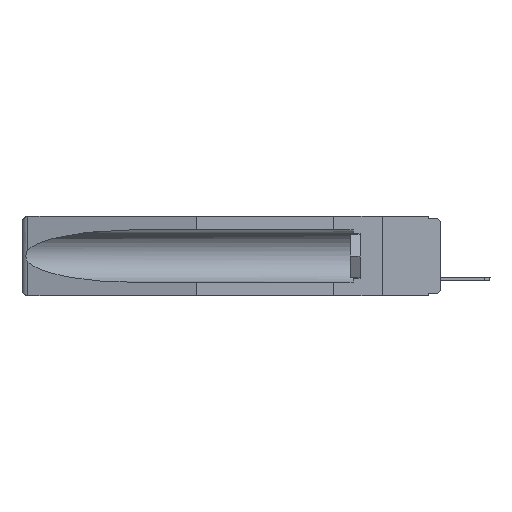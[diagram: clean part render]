
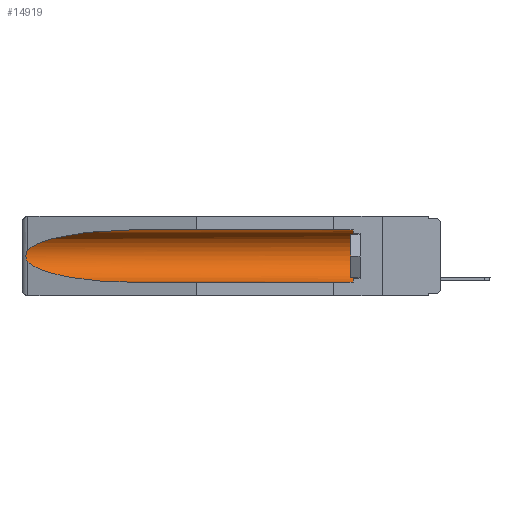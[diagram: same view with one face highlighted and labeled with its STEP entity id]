
A CAD part, left-side view. The second image highlights one B-rep face of the part: STEP entity #14919.
In plain terms, the highlighted cylindrical face has radius 2.857 mm (diameter 5.715 mm), a partial arc.
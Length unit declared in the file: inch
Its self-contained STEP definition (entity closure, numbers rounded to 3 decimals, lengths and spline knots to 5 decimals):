
#350 = DIRECTION ( 'NONE',  ( 0., 1., 0. ) ) ;
#384 = CARTESIAN_POINT ( 'NONE',  ( 0.155, 1.07973, -0.059 ) ) ;
#424 = ORIENTED_EDGE ( 'NONE', *, *, #5626, .T. ) ;
#513 = VERTEX_POINT ( 'NONE', #18364 ) ;
#762 = ORIENTED_EDGE ( 'NONE', *, *, #15672, .F. ) ;
#1241 = VECTOR ( 'NONE', #18341, 39.37008 ) ;
#1382 = VERTEX_POINT ( 'NONE', #384 ) ;
#1896 = CARTESIAN_POINT ( 'NONE',  ( 0.155, -0.30754, -0.059 ) ) ;
#2180 = CARTESIAN_POINT ( 'NONE',  ( 0.155, 0.126, -0.1715 ) ) ;
#2366 =( BOUNDED_CURVE ( )  B_SPLINE_CURVE ( 3, ( #6436, #12388, #16933, #3525 ),
 .UNSPECIFIED., .F., .F. ) 
 B_SPLINE_CURVE_WITH_KNOTS ( ( 4, 4 ),
 ( 4.71239, 6.08839 ),
 .UNSPECIFIED. ) 
 CURVE ( )  GEOMETRIC_REPRESENTATION_ITEM ( )  RATIONAL_B_SPLINE_CURVE ( ( 1., 0.848, 0.848, 1. ) ) 
 REPRESENTATION_ITEM ( '' )  );
#2823 = CIRCLE ( 'NONE', #17518, 0.1125 ) ;
#3043 = CARTESIAN_POINT ( 'NONE',  ( 0.26654, 1.53092, -0.15636 ) ) ;
#3142 = CARTESIAN_POINT ( 'NONE',  ( 0.2675, 1.53308, -0.16763 ) ) ;
#3234 = LINE ( 'NONE', #16838, #15283 ) ;
#3332 = CARTESIAN_POINT ( 'NONE',  ( 0.26537, 1.52718, -0.19328 ) ) ;
#3525 = CARTESIAN_POINT ( 'NONE',  ( 0.26537, 1.52718, -0.14972 ) ) ;
#3740 = DIRECTION ( 'NONE',  ( 0., 0., 1. ) ) ;
#4502 = CARTESIAN_POINT ( 'NONE',  ( 0.26597, 1.52961, -0.15275 ) ) ;
#4978 = CARTESIAN_POINT ( 'NONE',  ( 0.26597, 1.5296, -0.19026 ) ) ;
#5179 = DIRECTION ( 'NONE',  ( 0., -1., 0. ) ) ;
#5271 = CARTESIAN_POINT ( 'NONE',  ( 0.155, 1.07973, -0.284 ) ) ;
#5573 = CARTESIAN_POINT ( 'NONE',  ( 0.155, 0.126, -0.059 ) ) ;
#5626 = EDGE_CURVE ( 'NONE', #10328, #8989, #11929, .T. ) ;
#5648 = CARTESIAN_POINT ( 'NONE',  ( 0.21114, 1.30732, -0.284 ) ) ;
#6053 = CARTESIAN_POINT ( 'NONE',  ( 0.2673, 1.5327, -0.16383 ) ) ;
#6436 = CARTESIAN_POINT ( 'NONE',  ( 0.155, 1.07973, -0.059 ) ) ;
#6784 = ORIENTED_EDGE ( 'NONE', *, *, #7053, .T. ) ;
#7053 = EDGE_CURVE ( 'NONE', #8989, #15461, #15107, .T. ) ;
#7723 = ORIENTED_EDGE ( 'NONE', *, *, #17623, .T. ) ;
#7869 = VERTEX_POINT ( 'NONE', #5573 ) ;
#7901 = ORIENTED_EDGE ( 'NONE', *, *, #9360, .T. ) ;
#7943 = DIRECTION ( 'NONE',  ( 0., 0., 1. ) ) ;
#8288 = CARTESIAN_POINT ( 'NONE',  ( 0.25451, 1.48313, -0.24835 ) ) ;
#8975 = CARTESIAN_POINT ( 'NONE',  ( 0.2673, 1.53269, -0.17917 ) ) ;
#8989 = VERTEX_POINT ( 'NONE', #11730 ) ;
#9088 = EDGE_CURVE ( 'NONE', #7869, #1382, #12227, .T. ) ;
#9360 = EDGE_CURVE ( 'NONE', #513, #7869, #2823, .T. ) ;
#9414 = CYLINDRICAL_SURFACE ( 'NONE', #10843, 0.1125 ) ;
#9792 = EDGE_LOOP ( 'NONE', ( #7723, #424, #6784, #762, #7901, #17384 ) ) ;
#10120 = CARTESIAN_POINT ( 'NONE',  ( 0.26537, 1.52718, -0.19328 ) ) ;
#10328 = VERTEX_POINT ( 'NONE', #16973 ) ;
#10675 = CARTESIAN_POINT ( 'NONE',  ( 0.155, -0.30754, -0.1715 ) ) ;
#10843 = AXIS2_PLACEMENT_3D ( 'NONE', #10675, #350, #7943 ) ;
#11730 = CARTESIAN_POINT ( 'NONE',  ( 0.26537, 1.52718, -0.19328 ) ) ;
#11929 = B_SPLINE_CURVE_WITH_KNOTS ( 'NONE', 3,
 ( #17923, #4502, #3043, #6053, #3142, #15078, #8975, #12305, #4978, #3332 ),
 .UNSPECIFIED., .F., .F.,
 ( 4, 2, 2, 2, 4 ),
 ( 0., 0.00029, 0.00058, 0.00087, 0.00117 ),
 .UNSPECIFIED. ) ;
#12227 = LINE ( 'NONE', #1896, #1241 ) ;
#12305 = CARTESIAN_POINT ( 'NONE',  ( 0.26655, 1.53094, -0.18657 ) ) ;
#12388 = CARTESIAN_POINT ( 'NONE',  ( 0.21114, 1.30732, -0.059 ) ) ;
#14569 = CARTESIAN_POINT ( 'NONE',  ( 0.155, 1.07973, -0.284 ) ) ;
#14919 = ADVANCED_FACE ( 'NONE', ( #16889 ), #9414, .F. ) ;
#15078 = CARTESIAN_POINT ( 'NONE',  ( 0.2675, 1.53308, -0.17534 ) ) ;
#15107 =( BOUNDED_CURVE ( )  B_SPLINE_CURVE ( 3, ( #10120, #8288, #5648, #14569 ),
 .UNSPECIFIED., .F., .F. ) 
 B_SPLINE_CURVE_WITH_KNOTS ( ( 4, 4 ),
 ( 0.1948, 1.5708 ),
 .UNSPECIFIED. ) 
 CURVE ( )  GEOMETRIC_REPRESENTATION_ITEM ( )  RATIONAL_B_SPLINE_CURVE ( ( 1., 0.848, 0.848, 1. ) ) 
 REPRESENTATION_ITEM ( '' )  );
#15168 = DIRECTION ( 'NONE',  ( 0., 1., 0. ) ) ;
#15283 = VECTOR ( 'NONE', #15168, 39.37008 ) ;
#15461 = VERTEX_POINT ( 'NONE', #5271 ) ;
#15672 = EDGE_CURVE ( 'NONE', #513, #15461, #3234, .T. ) ;
#16838 = CARTESIAN_POINT ( 'NONE',  ( 0.155, -0.30754, -0.284 ) ) ;
#16889 = FACE_OUTER_BOUND ( 'NONE', #9792, .T. ) ;
#16933 = CARTESIAN_POINT ( 'NONE',  ( 0.25451, 1.48313, -0.09465 ) ) ;
#16973 = CARTESIAN_POINT ( 'NONE',  ( 0.26537, 1.52718, -0.14972 ) ) ;
#17384 = ORIENTED_EDGE ( 'NONE', *, *, #9088, .T. ) ;
#17518 = AXIS2_PLACEMENT_3D ( 'NONE', #2180, #5179, #3740 ) ;
#17623 = EDGE_CURVE ( 'NONE', #1382, #10328, #2366, .T. ) ;
#17923 = CARTESIAN_POINT ( 'NONE',  ( 0.26537, 1.52718, -0.14972 ) ) ;
#18341 = DIRECTION ( 'NONE',  ( 0., 1., 0. ) ) ;
#18364 = CARTESIAN_POINT ( 'NONE',  ( 0.155, 0.126, -0.284 ) ) ;
